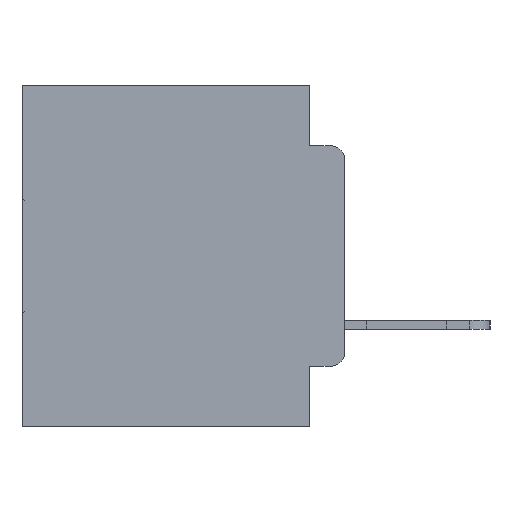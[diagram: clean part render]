
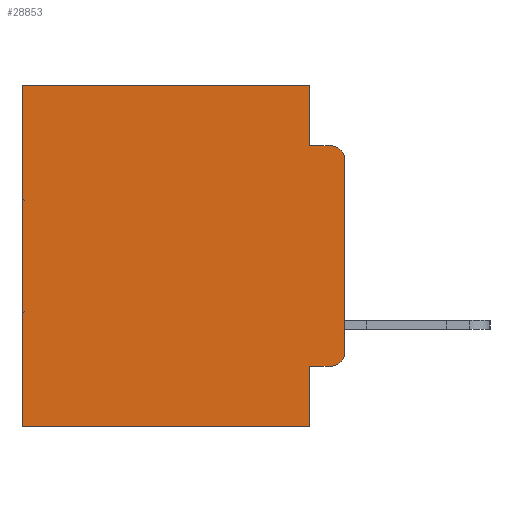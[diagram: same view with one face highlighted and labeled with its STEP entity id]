
A CAD part, left-side view. The second image highlights one B-rep face of the part: STEP entity #28853.
In plain terms, the highlighted planar face has unit normal (-1, 0, 0).
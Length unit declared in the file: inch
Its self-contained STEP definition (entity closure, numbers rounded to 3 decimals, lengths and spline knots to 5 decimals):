
#246 = VERTEX_POINT ( 'NONE', #14206 ) ;
#2358 = EDGE_CURVE ( 'NONE', #7585, #15252, #23806, .T. ) ;
#3833 = ORIENTED_EDGE ( 'NONE', *, *, #19654, .T. ) ;
#3854 = AXIS2_PLACEMENT_3D ( 'NONE', #28767, #19909, #20010 ) ;
#4281 = VECTOR ( 'NONE', #29549, 39.37008 ) ;
#4292 = LINE ( 'NONE', #9430, #23252 ) ;
#5425 = CIRCLE ( 'NONE', #22871, 0.02 ) ;
#5977 = CARTESIAN_POINT ( 'NONE',  ( 0.298, 0.02, -0.0885 ) ) ;
#6081 = VECTOR ( 'NONE', #9622, 39.37008 ) ;
#6570 = CARTESIAN_POINT ( 'NONE',  ( 0.298, 0.051, -0.0885 ) ) ;
#6770 = EDGE_LOOP ( 'NONE', ( #13770, #30801, #26412, #31135, #21046, #8101, #21318, #19810, #27462, #3833 ) ) ;
#7501 = VECTOR ( 'NONE', #12086, 39.37008 ) ;
#7585 = VERTEX_POINT ( 'NONE', #23641 ) ;
#8101 = ORIENTED_EDGE ( 'NONE', *, *, #18019, .T. ) ;
#8859 = CARTESIAN_POINT ( 'NONE',  ( 0.298, 0.051, 0. ) ) ;
#9213 = EDGE_CURVE ( 'NONE', #7585, #21554, #24630, .T. ) ;
#9374 = DIRECTION ( 'NONE',  ( 0., -1., 0. ) ) ;
#9430 = CARTESIAN_POINT ( 'NONE',  ( 0.298, 0.473, 0. ) ) ;
#9622 = DIRECTION ( 'NONE',  ( 0., 1., 0. ) ) ;
#9718 = VERTEX_POINT ( 'NONE', #8859 ) ;
#9851 = CARTESIAN_POINT ( 'NONE',  ( 0.298, 0.051, -0.5 ) ) ;
#10706 = PLANE ( 'NONE',  #29595 ) ;
#11195 = DIRECTION ( 'NONE',  ( 1., 0., 0. ) ) ;
#11909 = LINE ( 'NONE', #26576, #6081 ) ;
#12086 = DIRECTION ( 'NONE',  ( 0., -1., 0. ) ) ;
#12486 = LINE ( 'NONE', #16167, #18185 ) ;
#12562 = CARTESIAN_POINT ( 'NONE',  ( 0.298, 0., 0. ) ) ;
#13181 = EDGE_CURVE ( 'NONE', #30006, #18536, #21224, .T. ) ;
#13627 = FACE_OUTER_BOUND ( 'NONE', #6770, .T. ) ;
#13684 = CARTESIAN_POINT ( 'NONE',  ( 0.298, 0., -0.3915 ) ) ;
#13770 = ORIENTED_EDGE ( 'NONE', *, *, #9213, .F. ) ;
#14206 = CARTESIAN_POINT ( 'NONE',  ( 0.298, 0.051, -0.0885 ) ) ;
#15252 = VERTEX_POINT ( 'NONE', #5977 ) ;
#15729 = DIRECTION ( 'NONE',  ( 0., 1., 0. ) ) ;
#16167 = CARTESIAN_POINT ( 'NONE',  ( 0.298, 0.051, 0. ) ) ;
#17571 = VERTEX_POINT ( 'NONE', #9851 ) ;
#18019 = EDGE_CURVE ( 'NONE', #28459, #30249, #4292, .T. ) ;
#18185 = VECTOR ( 'NONE', #18545, 39.37008 ) ;
#18235 = VECTOR ( 'NONE', #26564, 39.37008 ) ;
#18437 = CARTESIAN_POINT ( 'NONE',  ( 0.298, 0.473, -0.5 ) ) ;
#18536 = VERTEX_POINT ( 'NONE', #19086 ) ;
#18545 = DIRECTION ( 'NONE',  ( 0., 0., -1. ) ) ;
#19086 = CARTESIAN_POINT ( 'NONE',  ( 0.298, 0.02, -0.4115 ) ) ;
#19654 = EDGE_CURVE ( 'NONE', #18536, #21554, #5425, .T. ) ;
#19810 = ORIENTED_EDGE ( 'NONE', *, *, #25987, .F. ) ;
#19909 = DIRECTION ( 'NONE',  ( -1., 0., 0. ) ) ;
#20010 = DIRECTION ( 'NONE',  ( 0., 0., -1. ) ) ;
#20439 = DIRECTION ( 'NONE',  ( 0., 0., -1. ) ) ;
#21046 = ORIENTED_EDGE ( 'NONE', *, *, #29901, .T. ) ;
#21224 = LINE ( 'NONE', #31225, #7501 ) ;
#21302 = DIRECTION ( 'NONE',  ( 0., 0., -1. ) ) ;
#21318 = ORIENTED_EDGE ( 'NONE', *, *, #24869, .F. ) ;
#21554 = VERTEX_POINT ( 'NONE', #13684 ) ;
#22135 = CARTESIAN_POINT ( 'NONE',  ( 0.298, 0., -0.5 ) ) ;
#22611 = VECTOR ( 'NONE', #9374, 39.37008 ) ;
#22871 = AXIS2_PLACEMENT_3D ( 'NONE', #28515, #25355, #21302 ) ;
#23252 = VECTOR ( 'NONE', #20439, 39.37008 ) ;
#23336 = VECTOR ( 'NONE', #15729, 39.37008 ) ;
#23363 = LINE ( 'NONE', #6570, #22611 ) ;
#23641 = CARTESIAN_POINT ( 'NONE',  ( 0.298, 0., -0.1085 ) ) ;
#23806 = CIRCLE ( 'NONE', #3854, 0.02 ) ;
#24488 = EDGE_CURVE ( 'NONE', #246, #15252, #23363, .T. ) ;
#24630 = LINE ( 'NONE', #29167, #18235 ) ;
#24869 = EDGE_CURVE ( 'NONE', #17571, #30249, #28578, .T. ) ;
#25355 = DIRECTION ( 'NONE',  ( -1., 0., 0. ) ) ;
#25987 = EDGE_CURVE ( 'NONE', #30006, #17571, #29187, .T. ) ;
#26412 = ORIENTED_EDGE ( 'NONE', *, *, #24488, .F. ) ;
#26564 = DIRECTION ( 'NONE',  ( 0., 0., -1. ) ) ;
#26576 = CARTESIAN_POINT ( 'NONE',  ( 0.298, 0., 0. ) ) ;
#26872 = DIRECTION ( 'NONE',  ( 0., 0., -1. ) ) ;
#27458 = EDGE_CURVE ( 'NONE', #9718, #246, #12486, .T. ) ;
#27462 = ORIENTED_EDGE ( 'NONE', *, *, #13181, .T. ) ;
#27773 = CARTESIAN_POINT ( 'NONE',  ( 0.298, 0.051, 0. ) ) ;
#28459 = VERTEX_POINT ( 'NONE', #29112 ) ;
#28515 = CARTESIAN_POINT ( 'NONE',  ( 0.298, 0.02, -0.3915 ) ) ;
#28578 = LINE ( 'NONE', #22135, #23336 ) ;
#28767 = CARTESIAN_POINT ( 'NONE',  ( 0.298, 0.02, -0.1085 ) ) ;
#28853 = ADVANCED_FACE ( 'NONE', ( #13627 ), #10706, .F. ) ;
#29112 = CARTESIAN_POINT ( 'NONE',  ( 0.298, 0.473, 0. ) ) ;
#29167 = CARTESIAN_POINT ( 'NONE',  ( 0.298, 0., 0. ) ) ;
#29187 = LINE ( 'NONE', #27773, #4281 ) ;
#29549 = DIRECTION ( 'NONE',  ( 0., 0., -1. ) ) ;
#29595 = AXIS2_PLACEMENT_3D ( 'NONE', #12562, #11195, #26872 ) ;
#29901 = EDGE_CURVE ( 'NONE', #9718, #28459, #11909, .T. ) ;
#30006 = VERTEX_POINT ( 'NONE', #31085 ) ;
#30249 = VERTEX_POINT ( 'NONE', #18437 ) ;
#30801 = ORIENTED_EDGE ( 'NONE', *, *, #2358, .T. ) ;
#31085 = CARTESIAN_POINT ( 'NONE',  ( 0.298, 0.051, -0.4115 ) ) ;
#31135 = ORIENTED_EDGE ( 'NONE', *, *, #27458, .F. ) ;
#31225 = CARTESIAN_POINT ( 'NONE',  ( 0.298, 0.051, -0.4115 ) ) ;
